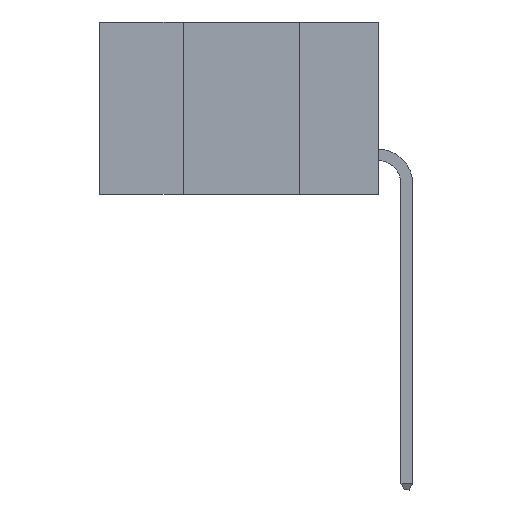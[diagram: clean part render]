
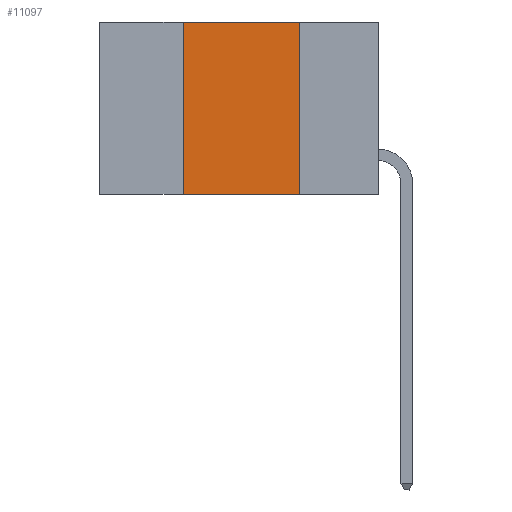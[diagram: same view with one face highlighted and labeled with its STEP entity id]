
A CAD part, left-side view. The second image highlights one B-rep face of the part: STEP entity #11097.
In plain terms, the highlighted planar face has unit normal (-1, 0, 0).
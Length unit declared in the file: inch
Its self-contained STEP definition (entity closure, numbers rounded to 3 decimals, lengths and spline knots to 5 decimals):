
#184 = EDGE_CURVE ( 'NONE', #3888, #837, #17905, .T. ) ;
#837 = VERTEX_POINT ( 'NONE', #12049 ) ;
#1897 = DIRECTION ( 'NONE',  ( 0., 0., 1. ) ) ;
#2352 = ORIENTED_EDGE ( 'NONE', *, *, #24798, .F. ) ;
#2736 = ORIENTED_EDGE ( 'NONE', *, *, #17767, .T. ) ;
#3886 = VECTOR ( 'NONE', #24425, 39.37008 ) ;
#3888 = VERTEX_POINT ( 'NONE', #18594 ) ;
#4028 = CARTESIAN_POINT ( 'NONE',  ( 0., 0.42, -0.37 ) ) ;
#5166 = PLANE ( 'NONE',  #9370 ) ;
#6433 = ORIENTED_EDGE ( 'NONE', *, *, #12915, .F. ) ;
#7239 = VERTEX_POINT ( 'NONE', #15404 ) ;
#8240 = EDGE_LOOP ( 'NONE', ( #6433, #11005, #2352, #2736 ) ) ;
#9370 = AXIS2_PLACEMENT_3D ( 'NONE', #20219, #24521, #11738 ) ;
#9421 = LINE ( 'NONE', #14703, #20078 ) ;
#9508 = CARTESIAN_POINT ( 'NONE',  ( 0., 0.6, -0.37 ) ) ;
#10121 = DIRECTION ( 'NONE',  ( 0., -1., 0. ) ) ;
#10562 = DIRECTION ( 'NONE',  ( 0., 0., -1. ) ) ;
#11005 = ORIENTED_EDGE ( 'NONE', *, *, #184, .F. ) ;
#11097 = ADVANCED_FACE ( 'NONE', ( #19483 ), #5166, .F. ) ;
#11738 = DIRECTION ( 'NONE',  ( 0., 0., -1. ) ) ;
#12049 = CARTESIAN_POINT ( 'NONE',  ( 0., 0.17, 0. ) ) ;
#12915 = EDGE_CURVE ( 'NONE', #837, #7239, #17057, .T. ) ;
#12996 = CARTESIAN_POINT ( 'NONE',  ( 0., 0.17, 0. ) ) ;
#14562 = VERTEX_POINT ( 'NONE', #4028 ) ;
#14595 = CARTESIAN_POINT ( 'NONE',  ( 0., 0.6, 0. ) ) ;
#14703 = CARTESIAN_POINT ( 'NONE',  ( 0., 0.42, 0. ) ) ;
#15404 = CARTESIAN_POINT ( 'NONE',  ( 0., 0.17, -0.37 ) ) ;
#15929 = VECTOR ( 'NONE', #10121, 39.37008 ) ;
#17057 = LINE ( 'NONE', #12996, #24733 ) ;
#17767 = EDGE_CURVE ( 'NONE', #14562, #7239, #22964, .T. ) ;
#17905 = LINE ( 'NONE', #14595, #15929 ) ;
#18594 = CARTESIAN_POINT ( 'NONE',  ( 0., 0.42, 0. ) ) ;
#19483 = FACE_OUTER_BOUND ( 'NONE', #8240, .T. ) ;
#20078 = VECTOR ( 'NONE', #1897, 39.37008 ) ;
#20219 = CARTESIAN_POINT ( 'NONE',  ( 0., 0.6, 0. ) ) ;
#22964 = LINE ( 'NONE', #9508, #3886 ) ;
#24425 = DIRECTION ( 'NONE',  ( 0., -1., 0. ) ) ;
#24521 = DIRECTION ( 'NONE',  ( 1., 0., 0. ) ) ;
#24733 = VECTOR ( 'NONE', #10562, 39.37008 ) ;
#24798 = EDGE_CURVE ( 'NONE', #14562, #3888, #9421, .T. ) ;
